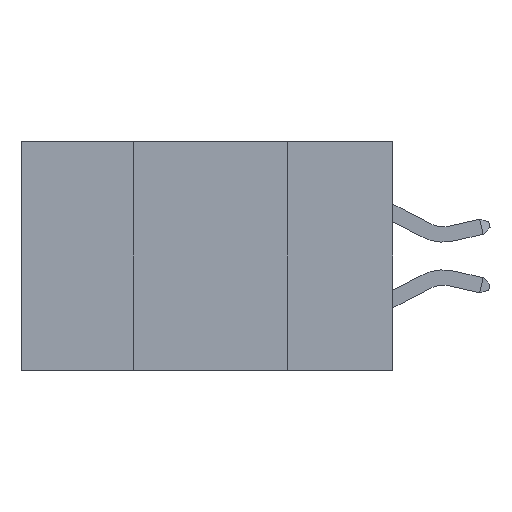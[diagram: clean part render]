
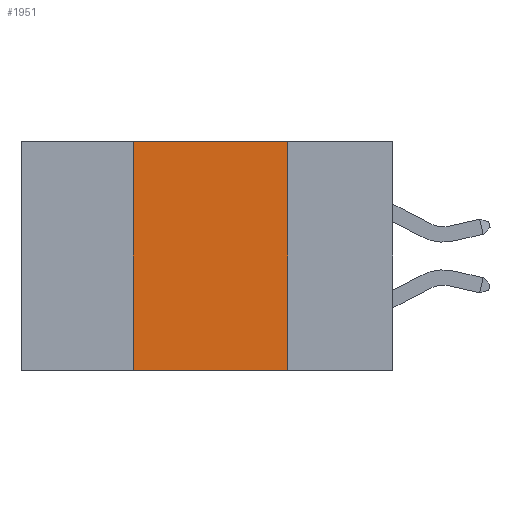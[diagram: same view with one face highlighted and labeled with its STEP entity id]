
A CAD part, left-side view. The second image highlights one B-rep face of the part: STEP entity #1951.
In plain terms, the highlighted planar face has unit normal (-1, 0, 0).
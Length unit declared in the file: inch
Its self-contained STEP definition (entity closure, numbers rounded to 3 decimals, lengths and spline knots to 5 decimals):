
#442 = DIRECTION ( 'NONE',  ( 0., -1., 0. ) ) ;
#512 = CARTESIAN_POINT ( 'NONE',  ( 0., 0.6, 0. ) ) ;
#1509 = ORIENTED_EDGE ( 'NONE', *, *, #3428, .F. ) ;
#1790 = EDGE_CURVE ( 'NONE', #9704, #4684, #4949, .T. ) ;
#1951 = ADVANCED_FACE ( 'NONE', ( #8045 ), #9043, .F. ) ;
#2142 = VERTEX_POINT ( 'NONE', #9287 ) ;
#2311 = ORIENTED_EDGE ( 'NONE', *, *, #10576, .F. ) ;
#3428 = EDGE_CURVE ( 'NONE', #2142, #8790, #6286, .T. ) ;
#4191 = CARTESIAN_POINT ( 'NONE',  ( 0., 0.17, -0.37 ) ) ;
#4216 = CARTESIAN_POINT ( 'NONE',  ( 0., 0.42, -0.37 ) ) ;
#4284 = VECTOR ( 'NONE', #6738, 39.37008 ) ;
#4684 = VERTEX_POINT ( 'NONE', #4191 ) ;
#4770 = VECTOR ( 'NONE', #10496, 39.37008 ) ;
#4840 = LINE ( 'NONE', #6688, #4770 ) ;
#4949 = LINE ( 'NONE', #7796, #4284 ) ;
#5161 = LINE ( 'NONE', #9825, #6752 ) ;
#5958 = DIRECTION ( 'NONE',  ( 0., 0., 1. ) ) ;
#6286 = LINE ( 'NONE', #512, #8646 ) ;
#6688 = CARTESIAN_POINT ( 'NONE',  ( 0., 0.17, 0. ) ) ;
#6718 = ORIENTED_EDGE ( 'NONE', *, *, #9561, .F. ) ;
#6738 = DIRECTION ( 'NONE',  ( 0., -1., 0. ) ) ;
#6752 = VECTOR ( 'NONE', #5958, 39.37008 ) ;
#7163 = DIRECTION ( 'NONE',  ( 0., 0., -1. ) ) ;
#7796 = CARTESIAN_POINT ( 'NONE',  ( 0., 0.6, -0.37 ) ) ;
#8045 = FACE_OUTER_BOUND ( 'NONE', #12237, .T. ) ;
#8061 = AXIS2_PLACEMENT_3D ( 'NONE', #11893, #11824, #7163 ) ;
#8646 = VECTOR ( 'NONE', #442, 39.37008 ) ;
#8790 = VERTEX_POINT ( 'NONE', #11443 ) ;
#9043 = PLANE ( 'NONE',  #8061 ) ;
#9287 = CARTESIAN_POINT ( 'NONE',  ( 0., 0.42, 0. ) ) ;
#9561 = EDGE_CURVE ( 'NONE', #8790, #4684, #4840, .T. ) ;
#9704 = VERTEX_POINT ( 'NONE', #4216 ) ;
#9825 = CARTESIAN_POINT ( 'NONE',  ( 0., 0.42, 0. ) ) ;
#10496 = DIRECTION ( 'NONE',  ( 0., 0., -1. ) ) ;
#10576 = EDGE_CURVE ( 'NONE', #9704, #2142, #5161, .T. ) ;
#11443 = CARTESIAN_POINT ( 'NONE',  ( 0., 0.17, 0. ) ) ;
#11824 = DIRECTION ( 'NONE',  ( 1., 0., 0. ) ) ;
#11893 = CARTESIAN_POINT ( 'NONE',  ( 0., 0.6, 0. ) ) ;
#11964 = ORIENTED_EDGE ( 'NONE', *, *, #1790, .T. ) ;
#12237 = EDGE_LOOP ( 'NONE', ( #6718, #1509, #2311, #11964 ) ) ;
